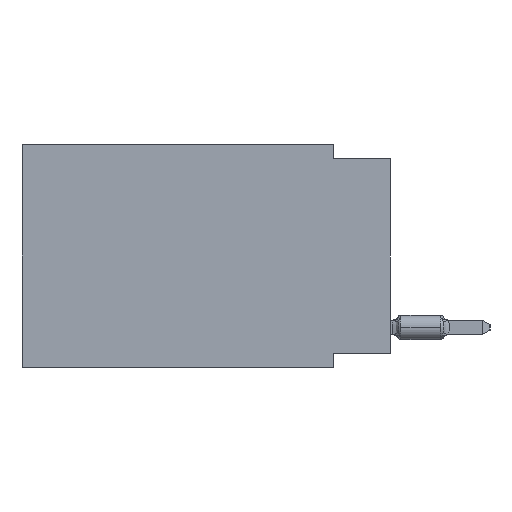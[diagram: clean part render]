
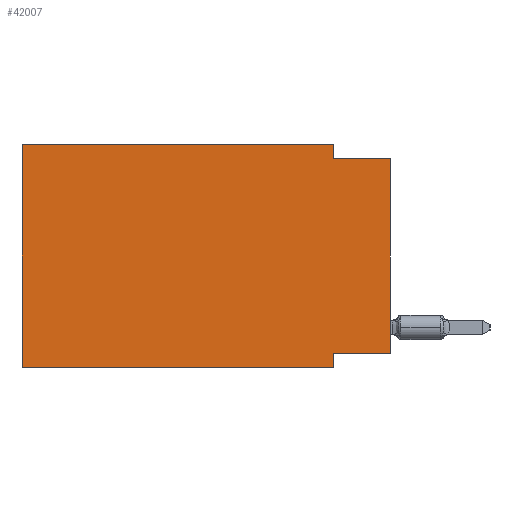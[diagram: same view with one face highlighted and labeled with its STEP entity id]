
A CAD part, left-side view. The second image highlights one B-rep face of the part: STEP entity #42007.
In plain terms, the highlighted planar face has unit normal (-1, 0, 0).
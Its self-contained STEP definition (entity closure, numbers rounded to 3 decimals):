
#21 = CARTESIAN_POINT ( 'NONE',  ( 0., 0., -0.635 ) ) ;
#163 = CARTESIAN_POINT ( 'NONE',  ( 0., 0., -9.271 ) ) ;
#2244 = VERTEX_POINT ( 'NONE', #37461 ) ;
#2862 = ORIENTED_EDGE ( 'NONE', *, *, #56253, .F. ) ;
#3949 = DIRECTION ( 'NONE',  ( 0., 1., 0. ) ) ;
#6115 = VECTOR ( 'NONE', #9192, 1000. ) ;
#6843 = DIRECTION ( 'NONE',  ( 1., 0., 0. ) ) ;
#7823 = LINE ( 'NONE', #10665, #49247 ) ;
#8191 = LINE ( 'NONE', #32823, #61916 ) ;
#9128 = EDGE_CURVE ( 'NONE', #51678, #64525, #23244, .T. ) ;
#9192 = DIRECTION ( 'NONE',  ( 0., -1., 0. ) ) ;
#10665 = CARTESIAN_POINT ( 'NONE',  ( 0., 16.383, -9.906 ) ) ;
#14643 = CARTESIAN_POINT ( 'NONE',  ( 0., 16.383, 0. ) ) ;
#14998 = ORIENTED_EDGE ( 'NONE', *, *, #51732, .T. ) ;
#17430 = DIRECTION ( 'NONE',  ( 0., 0., -1. ) ) ;
#19783 = LINE ( 'NONE', #14643, #6115 ) ;
#20404 = VERTEX_POINT ( 'NONE', #66967 ) ;
#20704 = CARTESIAN_POINT ( 'NONE',  ( 0., 16.383, 0. ) ) ;
#20891 = ORIENTED_EDGE ( 'NONE', *, *, #42243, .F. ) ;
#20893 = VECTOR ( 'NONE', #39586, 1000. ) ;
#21459 = CARTESIAN_POINT ( 'NONE',  ( 0., 0., -0.635 ) ) ;
#23244 = LINE ( 'NONE', #44111, #25750 ) ;
#23549 = ORIENTED_EDGE ( 'NONE', *, *, #66646, .T. ) ;
#23565 = VERTEX_POINT ( 'NONE', #51019 ) ;
#23985 = CARTESIAN_POINT ( 'NONE',  ( 0., 16.383, -9.906 ) ) ;
#24179 = LINE ( 'NONE', #65510, #20893 ) ;
#25750 = VECTOR ( 'NONE', #17430, 1000. ) ;
#27654 = CARTESIAN_POINT ( 'NONE',  ( 0., 2.54, 0. ) ) ;
#28918 = VERTEX_POINT ( 'NONE', #47975 ) ;
#29073 = AXIS2_PLACEMENT_3D ( 'NONE', #48211, #6843, #47526 ) ;
#29204 = LINE ( 'NONE', #21, #45546 ) ;
#31333 = EDGE_LOOP ( 'NONE', ( #23549, #48294, #37897, #20891, #60176, #14998, #2862, #55335 ) ) ;
#31447 = VECTOR ( 'NONE', #56945, 1000. ) ;
#32823 = CARTESIAN_POINT ( 'NONE',  ( 0., 2.54, -9.906 ) ) ;
#34248 = CARTESIAN_POINT ( 'NONE',  ( 0., 2.54, -0.635 ) ) ;
#34452 = VERTEX_POINT ( 'NONE', #21459 ) ;
#37461 = CARTESIAN_POINT ( 'NONE',  ( 0., 2.54, -9.271 ) ) ;
#37897 = ORIENTED_EDGE ( 'NONE', *, *, #9128, .F. ) ;
#39586 = DIRECTION ( 'NONE',  ( 0., 0., 1. ) ) ;
#42007 = ADVANCED_FACE ( 'NONE', ( #62884 ), #43426, .F. ) ;
#42243 = EDGE_CURVE ( 'NONE', #28918, #51678, #19783, .T. ) ;
#43426 = PLANE ( 'NONE',  #29073 ) ;
#44111 = CARTESIAN_POINT ( 'NONE',  ( 0., 2.54, 0. ) ) ;
#44949 = EDGE_CURVE ( 'NONE', #64525, #34452, #29204, .T. ) ;
#45546 = VECTOR ( 'NONE', #66990, 1000. ) ;
#45750 = EDGE_CURVE ( 'NONE', #53157, #28918, #46356, .T. ) ;
#46356 = LINE ( 'NONE', #20704, #31447 ) ;
#47526 = DIRECTION ( 'NONE',  ( 0., 0., -1. ) ) ;
#47975 = CARTESIAN_POINT ( 'NONE',  ( 0., 16.383, 0. ) ) ;
#48211 = CARTESIAN_POINT ( 'NONE',  ( 0., 16.383, 0. ) ) ;
#48294 = ORIENTED_EDGE ( 'NONE', *, *, #44949, .F. ) ;
#49187 = DIRECTION ( 'NONE',  ( 0., -1., 0. ) ) ;
#49247 = VECTOR ( 'NONE', #49187, 1000. ) ;
#50194 = EDGE_CURVE ( 'NONE', #23565, #2244, #52128, .T. ) ;
#51019 = CARTESIAN_POINT ( 'NONE',  ( 0., 0., -9.271 ) ) ;
#51678 = VERTEX_POINT ( 'NONE', #27654 ) ;
#51732 = EDGE_CURVE ( 'NONE', #53157, #20404, #7823, .T. ) ;
#52128 = LINE ( 'NONE', #163, #53583 ) ;
#53157 = VERTEX_POINT ( 'NONE', #23985 ) ;
#53583 = VECTOR ( 'NONE', #3949, 1000. ) ;
#53668 = DIRECTION ( 'NONE',  ( 0., 0., -1. ) ) ;
#55335 = ORIENTED_EDGE ( 'NONE', *, *, #50194, .F. ) ;
#56253 = EDGE_CURVE ( 'NONE', #2244, #20404, #8191, .T. ) ;
#56945 = DIRECTION ( 'NONE',  ( 0., 0., 1. ) ) ;
#60176 = ORIENTED_EDGE ( 'NONE', *, *, #45750, .F. ) ;
#61916 = VECTOR ( 'NONE', #53668, 1000. ) ;
#62884 = FACE_OUTER_BOUND ( 'NONE', #31333, .T. ) ;
#64525 = VERTEX_POINT ( 'NONE', #34248 ) ;
#65510 = CARTESIAN_POINT ( 'NONE',  ( 0., 0., 0. ) ) ;
#66646 = EDGE_CURVE ( 'NONE', #23565, #34452, #24179, .T. ) ;
#66967 = CARTESIAN_POINT ( 'NONE',  ( 0., 2.54, -9.906 ) ) ;
#66990 = DIRECTION ( 'NONE',  ( 0., -1., 0. ) ) ;
